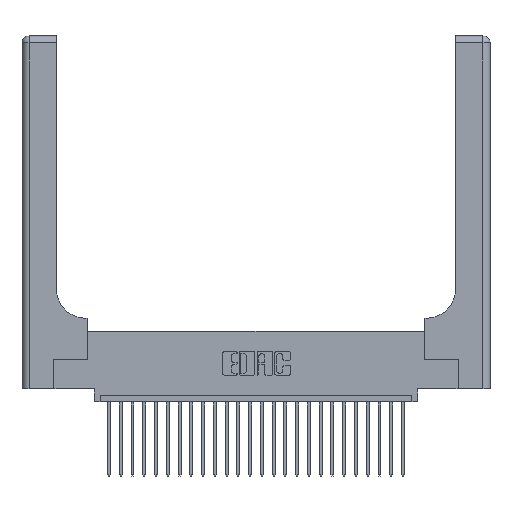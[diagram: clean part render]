
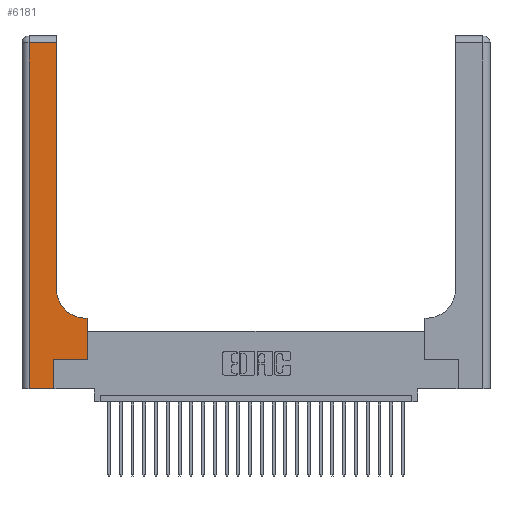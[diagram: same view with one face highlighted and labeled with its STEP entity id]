
A CAD part, top view. The second image highlights one B-rep face of the part: STEP entity #6181.
In plain terms, the highlighted planar face has unit normal (0, 0, 1).
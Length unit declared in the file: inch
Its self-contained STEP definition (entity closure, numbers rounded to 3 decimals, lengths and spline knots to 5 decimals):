
#303 = CARTESIAN_POINT ( 'NONE',  ( 0.5415, 0.85, 0.37 ) ) ;
#619 = CARTESIAN_POINT ( 'NONE',  ( 0.5585, 0.25, 0.37 ) ) ;
#1020 = ORIENTED_EDGE ( 'NONE', *, *, #7664, .T. ) ;
#1697 = LINE ( 'NONE', #619, #12139 ) ;
#2178 = CARTESIAN_POINT ( 'NONE',  ( 0., 3., 0.37 ) ) ;
#2272 = DIRECTION ( 'NONE',  ( 0., 0., -1. ) ) ;
#2863 = VECTOR ( 'NONE', #23068, 39.37008 ) ;
#2971 = VERTEX_POINT ( 'NONE', #22867 ) ;
#3455 = VERTEX_POINT ( 'NONE', #14386 ) ;
#3516 = CIRCLE ( 'NONE', #22180, 0.25 ) ;
#3597 = DIRECTION ( 'NONE',  ( 1., 0., 0. ) ) ;
#3815 = AXIS2_PLACEMENT_3D ( 'NONE', #2178, #2272, #22988 ) ;
#3929 = LINE ( 'NONE', #11789, #4598 ) ;
#4160 = CARTESIAN_POINT ( 'NONE',  ( 0.269, 0.25, 0.37 ) ) ;
#4476 = DIRECTION ( 'NONE',  ( -1., 0., 0. ) ) ;
#4598 = VECTOR ( 'NONE', #11970, 39.37008 ) ;
#4732 = VERTEX_POINT ( 'NONE', #23613 ) ;
#5474 = FACE_OUTER_BOUND ( 'NONE', #9540, .T. ) ;
#5794 = CARTESIAN_POINT ( 'NONE',  ( 0.5415, 0.6, 0.37 ) ) ;
#6181 = ADVANCED_FACE ( 'NONE', ( #5474 ), #10370, .F. ) ;
#6729 = VERTEX_POINT ( 'NONE', #8513 ) ;
#7330 = LINE ( 'NONE', #9043, #25978 ) ;
#7664 = EDGE_CURVE ( 'NONE', #9172, #4732, #21387, .T. ) ;
#7791 = ORIENTED_EDGE ( 'NONE', *, *, #11417, .T. ) ;
#7795 = EDGE_CURVE ( 'NONE', #22905, #19169, #13259, .T. ) ;
#8500 = CARTESIAN_POINT ( 'NONE',  ( 0.2915, 0.6, 0.37 ) ) ;
#8513 = CARTESIAN_POINT ( 'NONE',  ( 0.2915, 2.94, 0.37 ) ) ;
#8679 = DIRECTION ( 'NONE',  ( 0., 1., 0. ) ) ;
#9043 = CARTESIAN_POINT ( 'NONE',  ( 0.2915, 3., 0.37 ) ) ;
#9167 = VECTOR ( 'NONE', #3597, 39.37008 ) ;
#9172 = VERTEX_POINT ( 'NONE', #25506 ) ;
#9346 = EDGE_CURVE ( 'NONE', #20349, #22905, #1697, .T. ) ;
#9540 = EDGE_LOOP ( 'NONE', ( #14911, #10881, #12375, #11515, #1020, #7791, #19777, #11000, #19319 ) ) ;
#9653 = EDGE_CURVE ( 'NONE', #6729, #3455, #24214, .T. ) ;
#10037 = EDGE_CURVE ( 'NONE', #3455, #2971, #3929, .T. ) ;
#10370 = PLANE ( 'NONE',  #3815 ) ;
#10881 = ORIENTED_EDGE ( 'NONE', *, *, #9653, .T. ) ;
#11000 = ORIENTED_EDGE ( 'NONE', *, *, #7795, .T. ) ;
#11342 = DIRECTION ( 'NONE',  ( 0., 1., 0. ) ) ;
#11417 = EDGE_CURVE ( 'NONE', #4732, #20349, #20789, .T. ) ;
#11515 = ORIENTED_EDGE ( 'NONE', *, *, #25143, .T. ) ;
#11769 = CARTESIAN_POINT ( 'NONE',  ( 0.5585, 0.6, 0.37 ) ) ;
#11789 = CARTESIAN_POINT ( 'NONE',  ( 0.06, 3., 0.37 ) ) ;
#11970 = DIRECTION ( 'NONE',  ( 0., -1., 0. ) ) ;
#12139 = VECTOR ( 'NONE', #11342, 39.37008 ) ;
#12242 = VECTOR ( 'NONE', #8679, 39.37008 ) ;
#12375 = ORIENTED_EDGE ( 'NONE', *, *, #10037, .T. ) ;
#13259 = LINE ( 'NONE', #8500, #16789 ) ;
#13356 = EDGE_CURVE ( 'NONE', #16218, #6729, #7330, .T. ) ;
#14386 = CARTESIAN_POINT ( 'NONE',  ( 0.06, 2.94, 0.37 ) ) ;
#14895 = DIRECTION ( 'NONE',  ( 0., 0., -1. ) ) ;
#14911 = ORIENTED_EDGE ( 'NONE', *, *, #13356, .T. ) ;
#16218 = VERTEX_POINT ( 'NONE', #18159 ) ;
#16789 = VECTOR ( 'NONE', #22948, 39.37008 ) ;
#17241 = CARTESIAN_POINT ( 'NONE',  ( 0.269, 0., 0.37 ) ) ;
#17261 = EDGE_CURVE ( 'NONE', #19169, #16218, #3516, .T. ) ;
#17357 = DIRECTION ( 'NONE',  ( 0., 1., 0. ) ) ;
#18159 = CARTESIAN_POINT ( 'NONE',  ( 0.2915, 0.85, 0.37 ) ) ;
#19169 = VERTEX_POINT ( 'NONE', #5794 ) ;
#19319 = ORIENTED_EDGE ( 'NONE', *, *, #17261, .T. ) ;
#19624 = LINE ( 'NONE', #22241, #9167 ) ;
#19636 = VECTOR ( 'NONE', #4476, 39.37008 ) ;
#19777 = ORIENTED_EDGE ( 'NONE', *, *, #9346, .T. ) ;
#20349 = VERTEX_POINT ( 'NONE', #24267 ) ;
#20789 = LINE ( 'NONE', #4160, #2863 ) ;
#21258 = CARTESIAN_POINT ( 'NONE',  ( 0., 2.94, 0.37 ) ) ;
#21387 = LINE ( 'NONE', #17241, #12242 ) ;
#22180 = AXIS2_PLACEMENT_3D ( 'NONE', #303, #14895, #25484 ) ;
#22241 = CARTESIAN_POINT ( 'NONE',  ( 0., 0., 0.37 ) ) ;
#22867 = CARTESIAN_POINT ( 'NONE',  ( 0.06, 0., 0.37 ) ) ;
#22905 = VERTEX_POINT ( 'NONE', #11769 ) ;
#22948 = DIRECTION ( 'NONE',  ( -1., 0., 0. ) ) ;
#22988 = DIRECTION ( 'NONE',  ( -1., 0., 0. ) ) ;
#23068 = DIRECTION ( 'NONE',  ( 1., 0., 0. ) ) ;
#23613 = CARTESIAN_POINT ( 'NONE',  ( 0.269, 0.25, 0.37 ) ) ;
#24214 = LINE ( 'NONE', #21258, #19636 ) ;
#24267 = CARTESIAN_POINT ( 'NONE',  ( 0.5585, 0.25, 0.37 ) ) ;
#25143 = EDGE_CURVE ( 'NONE', #2971, #9172, #19624, .T. ) ;
#25484 = DIRECTION ( 'NONE',  ( 1., 0., 0. ) ) ;
#25506 = CARTESIAN_POINT ( 'NONE',  ( 0.269, 0., 0.37 ) ) ;
#25978 = VECTOR ( 'NONE', #17357, 39.37008 ) ;
